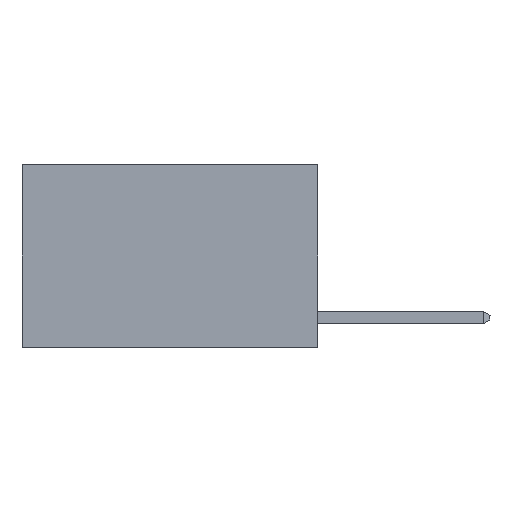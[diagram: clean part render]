
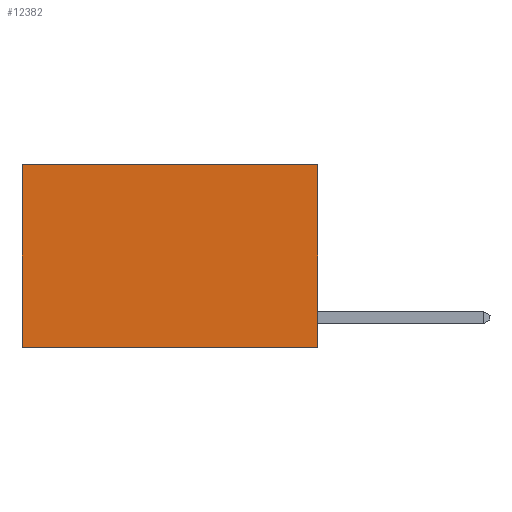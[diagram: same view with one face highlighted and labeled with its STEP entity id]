
A CAD part, left-side view. The second image highlights one B-rep face of the part: STEP entity #12382.
In plain terms, the highlighted planar face has unit normal (-1, 0, 0).
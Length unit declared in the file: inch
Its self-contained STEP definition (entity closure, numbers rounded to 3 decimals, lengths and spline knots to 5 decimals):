
#565 = LINE ( 'NONE', #11538, #9793 ) ;
#689 = DIRECTION ( 'NONE',  ( 0., 1., 0. ) ) ;
#1676 = DIRECTION ( 'NONE',  ( 0., 0., -1. ) ) ;
#2347 = CARTESIAN_POINT ( 'NONE',  ( 0.2625, 0.6, -0.37 ) ) ;
#2461 = LINE ( 'NONE', #3626, #5878 ) ;
#2510 = VERTEX_POINT ( 'NONE', #5593 ) ;
#2522 = VECTOR ( 'NONE', #10797, 39.37008 ) ;
#2811 = DIRECTION ( 'NONE',  ( 1., 0., 0. ) ) ;
#3578 = VERTEX_POINT ( 'NONE', #7821 ) ;
#3626 = CARTESIAN_POINT ( 'NONE',  ( 0.2625, 0.6, 0. ) ) ;
#3830 = EDGE_CURVE ( 'NONE', #8680, #10856, #565, .T. ) ;
#3937 = CARTESIAN_POINT ( 'NONE',  ( 0.2625, 0., 0. ) ) ;
#4212 = AXIS2_PLACEMENT_3D ( 'NONE', #4483, #2811, #4605 ) ;
#4467 = CARTESIAN_POINT ( 'NONE',  ( 0.2625, 0., 0. ) ) ;
#4483 = CARTESIAN_POINT ( 'NONE',  ( 0.2625, 0., 0. ) ) ;
#4605 = DIRECTION ( 'NONE',  ( 0., 0., -1. ) ) ;
#4653 = DIRECTION ( 'NONE',  ( 0., 1., 0. ) ) ;
#5593 = CARTESIAN_POINT ( 'NONE',  ( 0.2625, 0.6, 0. ) ) ;
#5878 = VECTOR ( 'NONE', #1676, 39.37008 ) ;
#6285 = ORIENTED_EDGE ( 'NONE', *, *, #3830, .F. ) ;
#6405 = ORIENTED_EDGE ( 'NONE', *, *, #8333, .F. ) ;
#6504 = ORIENTED_EDGE ( 'NONE', *, *, #11409, .T. ) ;
#7522 = ORIENTED_EDGE ( 'NONE', *, *, #11499, .T. ) ;
#7821 = CARTESIAN_POINT ( 'NONE',  ( 0.2625, 0., 0. ) ) ;
#8333 = EDGE_CURVE ( 'NONE', #3578, #8680, #10672, .T. ) ;
#8358 = CARTESIAN_POINT ( 'NONE',  ( 0.2625, 0., -0.37 ) ) ;
#8680 = VERTEX_POINT ( 'NONE', #8358 ) ;
#9793 = VECTOR ( 'NONE', #689, 39.37008 ) ;
#10440 = FACE_OUTER_BOUND ( 'NONE', #10808, .T. ) ;
#10672 = LINE ( 'NONE', #3937, #2522 ) ;
#10797 = DIRECTION ( 'NONE',  ( 0., 0., -1. ) ) ;
#10808 = EDGE_LOOP ( 'NONE', ( #6504, #6285, #6405, #7522 ) ) ;
#10856 = VERTEX_POINT ( 'NONE', #2347 ) ;
#11241 = VECTOR ( 'NONE', #4653, 39.37008 ) ;
#11409 = EDGE_CURVE ( 'NONE', #2510, #10856, #2461, .T. ) ;
#11454 = LINE ( 'NONE', #4467, #11241 ) ;
#11499 = EDGE_CURVE ( 'NONE', #3578, #2510, #11454, .T. ) ;
#11538 = CARTESIAN_POINT ( 'NONE',  ( 0.2625, 0., -0.37 ) ) ;
#12312 = PLANE ( 'NONE',  #4212 ) ;
#12382 = ADVANCED_FACE ( 'NONE', ( #10440 ), #12312, .F. ) ;
